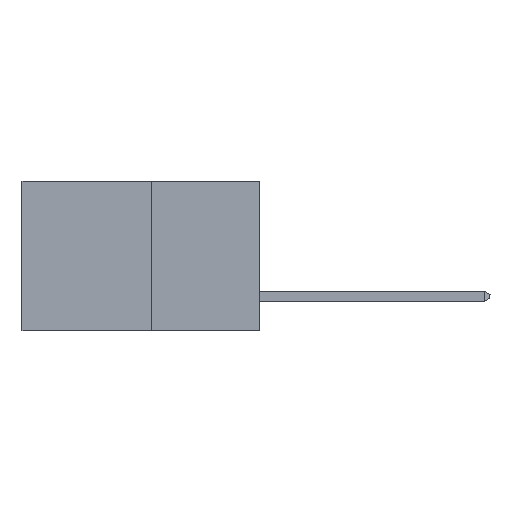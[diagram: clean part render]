
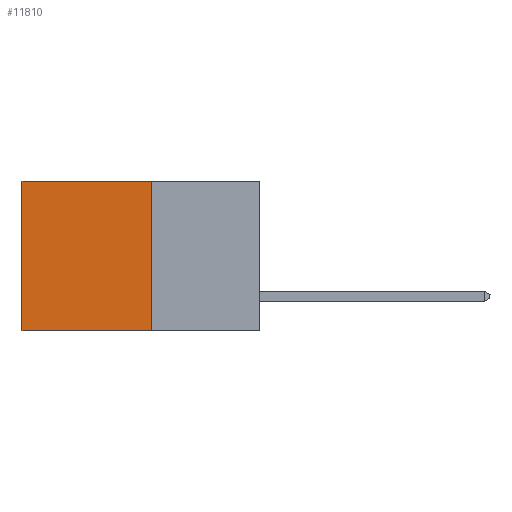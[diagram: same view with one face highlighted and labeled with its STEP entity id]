
A CAD part, left-side view. The second image highlights one B-rep face of the part: STEP entity #11810.
In plain terms, the highlighted planar face has unit normal (-1, 0, 0).
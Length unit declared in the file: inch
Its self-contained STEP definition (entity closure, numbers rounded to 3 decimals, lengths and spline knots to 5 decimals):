
#210 = LINE ( 'NONE', #11200, #3219 ) ;
#329 = VERTEX_POINT ( 'NONE', #11210 ) ;
#605 = EDGE_CURVE ( 'NONE', #1391, #11562, #7702, .T. ) ;
#881 = ORIENTED_EDGE ( 'NONE', *, *, #1047, .F. ) ;
#1047 = EDGE_CURVE ( 'NONE', #1391, #329, #12385, .T. ) ;
#1391 = VERTEX_POINT ( 'NONE', #2434 ) ;
#1506 = EDGE_CURVE ( 'NONE', #11562, #14001, #210, .T. ) ;
#1581 = AXIS2_PLACEMENT_3D ( 'NONE', #3160, #11038, #4309 ) ;
#1824 = FACE_OUTER_BOUND ( 'NONE', #5939, .T. ) ;
#1871 = ORIENTED_EDGE ( 'NONE', *, *, #1506, .T. ) ;
#2030 = DIRECTION ( 'NONE',  ( 0., 1., 0. ) ) ;
#2434 = CARTESIAN_POINT ( 'NONE',  ( 0.277, 0.27, 0. ) ) ;
#3160 = CARTESIAN_POINT ( 'NONE',  ( 0.277, 0.27, -0.37 ) ) ;
#3219 = VECTOR ( 'NONE', #13356, 39.37008 ) ;
#4138 = VECTOR ( 'NONE', #12501, 39.37008 ) ;
#4309 = DIRECTION ( 'NONE',  ( 0., 0., -1. ) ) ;
#4698 = VECTOR ( 'NONE', #11888, 39.37008 ) ;
#5939 = EDGE_LOOP ( 'NONE', ( #1871, #14560, #881, #10832 ) ) ;
#7702 = LINE ( 'NONE', #10565, #4698 ) ;
#8144 = LINE ( 'NONE', #10030, #13726 ) ;
#8763 = PLANE ( 'NONE',  #1581 ) ;
#10030 = CARTESIAN_POINT ( 'NONE',  ( 0.277, 0.27, -0.37 ) ) ;
#10565 = CARTESIAN_POINT ( 'NONE',  ( 0.277, 0.27, 0. ) ) ;
#10832 = ORIENTED_EDGE ( 'NONE', *, *, #605, .T. ) ;
#11038 = DIRECTION ( 'NONE',  ( 1., 0., 0. ) ) ;
#11115 = EDGE_CURVE ( 'NONE', #329, #14001, #8144, .T. ) ;
#11200 = CARTESIAN_POINT ( 'NONE',  ( 0.277, 0.59, -0.37 ) ) ;
#11210 = CARTESIAN_POINT ( 'NONE',  ( 0.277, 0.27, -0.37 ) ) ;
#11562 = VERTEX_POINT ( 'NONE', #12865 ) ;
#11810 = ADVANCED_FACE ( 'NONE', ( #1824 ), #8763, .F. ) ;
#11888 = DIRECTION ( 'NONE',  ( 0., 1., 0. ) ) ;
#12385 = LINE ( 'NONE', #12452, #4138 ) ;
#12452 = CARTESIAN_POINT ( 'NONE',  ( 0.277, 0.27, -0.37 ) ) ;
#12501 = DIRECTION ( 'NONE',  ( 0., 0., -1. ) ) ;
#12865 = CARTESIAN_POINT ( 'NONE',  ( 0.277, 0.59, 0. ) ) ;
#12938 = CARTESIAN_POINT ( 'NONE',  ( 0.277, 0.59, -0.37 ) ) ;
#13356 = DIRECTION ( 'NONE',  ( 0., 0., -1. ) ) ;
#13726 = VECTOR ( 'NONE', #2030, 39.37008 ) ;
#14001 = VERTEX_POINT ( 'NONE', #12938 ) ;
#14560 = ORIENTED_EDGE ( 'NONE', *, *, #11115, .F. ) ;
